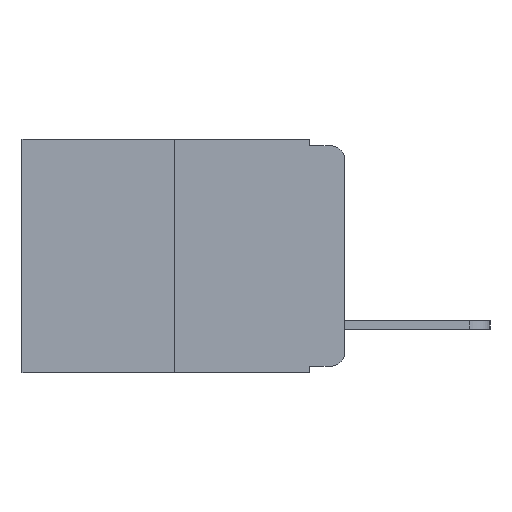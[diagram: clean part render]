
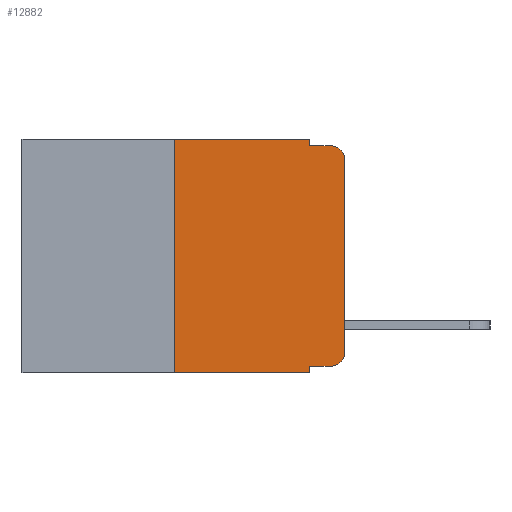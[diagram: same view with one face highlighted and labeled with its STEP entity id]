
A CAD part, left-side view. The second image highlights one B-rep face of the part: STEP entity #12882.
In plain terms, the highlighted planar face has unit normal (-1, 0, 0).
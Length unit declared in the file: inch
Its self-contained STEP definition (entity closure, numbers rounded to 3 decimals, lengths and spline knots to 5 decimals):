
#157 = EDGE_CURVE ( 'NONE', #4467, #13407, #3947, .T. ) ;
#316 = CARTESIAN_POINT ( 'NONE',  ( 0., 0.051, -0.01 ) ) ;
#401 = VERTEX_POINT ( 'NONE', #10267 ) ;
#434 = ORIENTED_EDGE ( 'NONE', *, *, #17579, .T. ) ;
#476 = CARTESIAN_POINT ( 'NONE',  ( 0., 0.02, -0.313 ) ) ;
#719 = DIRECTION ( 'NONE',  ( -1., 0., 0. ) ) ;
#759 = EDGE_LOOP ( 'NONE', ( #434, #6502, #2887, #3114, #17358, #12512, #2718, #3439, #3870, #4008 ) ) ;
#1645 = VECTOR ( 'NONE', #10329, 39.37008 ) ;
#1757 = LINE ( 'NONE', #8949, #16766 ) ;
#1767 = AXIS2_PLACEMENT_3D ( 'NONE', #9954, #719, #11396 ) ;
#1770 = CARTESIAN_POINT ( 'NONE',  ( 0., 0.25, 0. ) ) ;
#2169 = CARTESIAN_POINT ( 'NONE',  ( 0., 0.25, -0.343 ) ) ;
#2202 = DIRECTION ( 'NONE',  ( 0., 0., -1. ) ) ;
#2231 = LINE ( 'NONE', #16856, #17153 ) ;
#2247 = VECTOR ( 'NONE', #15117, 39.37008 ) ;
#2313 = DIRECTION ( 'NONE',  ( 1., 0., 0. ) ) ;
#2689 = DIRECTION ( 'NONE',  ( 0., 0., 1. ) ) ;
#2692 = VERTEX_POINT ( 'NONE', #2169 ) ;
#2718 = ORIENTED_EDGE ( 'NONE', *, *, #8293, .T. ) ;
#2887 = ORIENTED_EDGE ( 'NONE', *, *, #10298, .F. ) ;
#3114 = ORIENTED_EDGE ( 'NONE', *, *, #157, .F. ) ;
#3160 = CARTESIAN_POINT ( 'NONE',  ( 0., 0.051, -0.343 ) ) ;
#3439 = ORIENTED_EDGE ( 'NONE', *, *, #8158, .F. ) ;
#3544 = VERTEX_POINT ( 'NONE', #1770 ) ;
#3658 = DIRECTION ( 'NONE',  ( 0., 0., -1. ) ) ;
#3870 = ORIENTED_EDGE ( 'NONE', *, *, #7831, .T. ) ;
#3947 = LINE ( 'NONE', #9714, #18528 ) ;
#4008 = ORIENTED_EDGE ( 'NONE', *, *, #16968, .T. ) ;
#4071 = EDGE_CURVE ( 'NONE', #2692, #3544, #1757, .T. ) ;
#4467 = VERTEX_POINT ( 'NONE', #9962 ) ;
#5028 = FACE_OUTER_BOUND ( 'NONE', #759, .T. ) ;
#5107 = LINE ( 'NONE', #14735, #12417 ) ;
#5162 = VERTEX_POINT ( 'NONE', #3160 ) ;
#5658 = EDGE_CURVE ( 'NONE', #3544, #4467, #18269, .T. ) ;
#6502 = ORIENTED_EDGE ( 'NONE', *, *, #12250, .T. ) ;
#7606 = DIRECTION ( 'NONE',  ( 0., -1., 0. ) ) ;
#7831 = EDGE_CURVE ( 'NONE', #10333, #12059, #17167, .T. ) ;
#8158 = EDGE_CURVE ( 'NONE', #10333, #5162, #18776, .T. ) ;
#8171 = VECTOR ( 'NONE', #18508, 39.37008 ) ;
#8293 = EDGE_CURVE ( 'NONE', #2692, #5162, #2231, .T. ) ;
#8338 = CARTESIAN_POINT ( 'NONE',  ( 0., 0.473, 0. ) ) ;
#8949 = CARTESIAN_POINT ( 'NONE',  ( 0., 0.25, 0. ) ) ;
#9179 = AXIS2_PLACEMENT_3D ( 'NONE', #8338, #2313, #12718 ) ;
#9714 = CARTESIAN_POINT ( 'NONE',  ( 0., 0.051, 0. ) ) ;
#9954 = CARTESIAN_POINT ( 'NONE',  ( 0., 0.02, -0.03 ) ) ;
#9962 = CARTESIAN_POINT ( 'NONE',  ( 0., 0.051, 0. ) ) ;
#9999 = CARTESIAN_POINT ( 'NONE',  ( 0., 0.051, -0.333 ) ) ;
#10267 = CARTESIAN_POINT ( 'NONE',  ( 0., 0., -0.03 ) ) ;
#10298 = EDGE_CURVE ( 'NONE', #13407, #15877, #11090, .T. ) ;
#10329 = DIRECTION ( 'NONE',  ( 0., -1., 0. ) ) ;
#10333 = VERTEX_POINT ( 'NONE', #9999 ) ;
#10459 = CARTESIAN_POINT ( 'NONE',  ( 0., 0.051, -0.01 ) ) ;
#10846 = CARTESIAN_POINT ( 'NONE',  ( 0., 0.473, 0. ) ) ;
#10917 = CARTESIAN_POINT ( 'NONE',  ( 0., 0.02, -0.333 ) ) ;
#11090 = LINE ( 'NONE', #10459, #1645 ) ;
#11202 = DIRECTION ( 'NONE',  ( -1., 0., 0. ) ) ;
#11307 = PLANE ( 'NONE',  #9179 ) ;
#11396 = DIRECTION ( 'NONE',  ( 0., 0., -1. ) ) ;
#11566 = CIRCLE ( 'NONE', #17974, 0.02 ) ;
#12059 = VERTEX_POINT ( 'NONE', #10917 ) ;
#12164 = CIRCLE ( 'NONE', #1767, 0.02 ) ;
#12250 = EDGE_CURVE ( 'NONE', #401, #15877, #12164, .T. ) ;
#12417 = VECTOR ( 'NONE', #16117, 39.37008 ) ;
#12512 = ORIENTED_EDGE ( 'NONE', *, *, #4071, .F. ) ;
#12718 = DIRECTION ( 'NONE',  ( 0., 0., -1. ) ) ;
#12882 = ADVANCED_FACE ( 'NONE', ( #5028 ), #11307, .F. ) ;
#13407 = VERTEX_POINT ( 'NONE', #316 ) ;
#14028 = CARTESIAN_POINT ( 'NONE',  ( 0., 0.051, -0.333 ) ) ;
#14735 = CARTESIAN_POINT ( 'NONE',  ( 0., 0., 0. ) ) ;
#14758 = VECTOR ( 'NONE', #7606, 39.37008 ) ;
#14888 = CARTESIAN_POINT ( 'NONE',  ( 0., 0., -0.313 ) ) ;
#15117 = DIRECTION ( 'NONE',  ( 0., -1., 0. ) ) ;
#15195 = CARTESIAN_POINT ( 'NONE',  ( 0., 0.02, -0.01 ) ) ;
#15877 = VERTEX_POINT ( 'NONE', #15195 ) ;
#16117 = DIRECTION ( 'NONE',  ( 0., 0., 1. ) ) ;
#16766 = VECTOR ( 'NONE', #2689, 39.37008 ) ;
#16841 = DIRECTION ( 'NONE',  ( 0., -1., 0. ) ) ;
#16856 = CARTESIAN_POINT ( 'NONE',  ( 0., 0.473, -0.343 ) ) ;
#16968 = EDGE_CURVE ( 'NONE', #12059, #18684, #11566, .T. ) ;
#17153 = VECTOR ( 'NONE', #16841, 39.37008 ) ;
#17167 = LINE ( 'NONE', #14028, #2247 ) ;
#17358 = ORIENTED_EDGE ( 'NONE', *, *, #5658, .F. ) ;
#17579 = EDGE_CURVE ( 'NONE', #18684, #401, #5107, .T. ) ;
#17974 = AXIS2_PLACEMENT_3D ( 'NONE', #476, #11202, #2202 ) ;
#18269 = LINE ( 'NONE', #10846, #14758 ) ;
#18397 = CARTESIAN_POINT ( 'NONE',  ( 0., 0.051, 0. ) ) ;
#18508 = DIRECTION ( 'NONE',  ( 0., 0., -1. ) ) ;
#18528 = VECTOR ( 'NONE', #3658, 39.37008 ) ;
#18684 = VERTEX_POINT ( 'NONE', #14888 ) ;
#18776 = LINE ( 'NONE', #18397, #8171 ) ;
